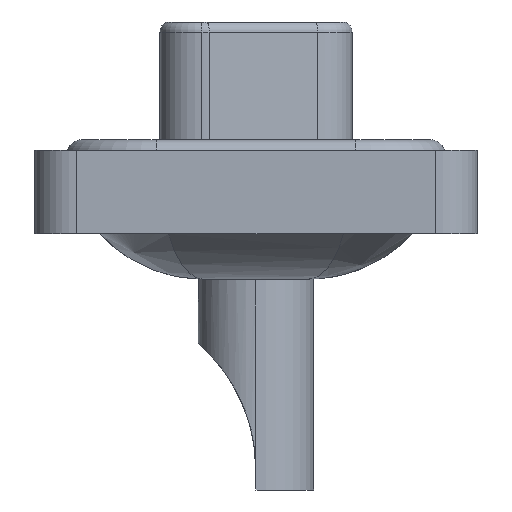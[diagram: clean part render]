
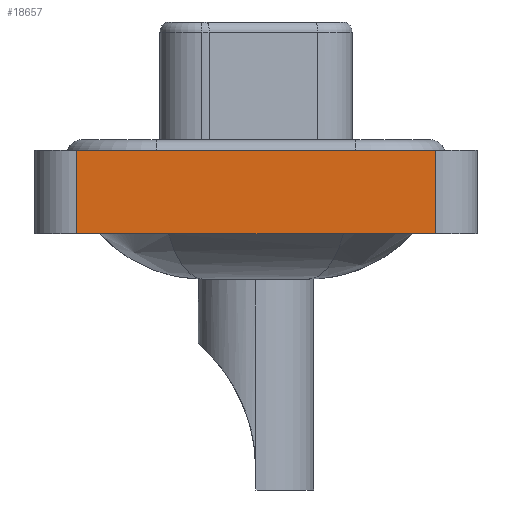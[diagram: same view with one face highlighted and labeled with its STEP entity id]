
A CAD part, left-side view. The second image highlights one B-rep face of the part: STEP entity #18657.
In plain terms, the highlighted planar face has unit normal (-1, 0, 0).
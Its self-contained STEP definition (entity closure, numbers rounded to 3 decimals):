
#525 = CARTESIAN_POINT ( 'NONE',  ( -7.3, 8.55, -3.6 ) ) ;
#1824 = DIRECTION ( 'NONE',  ( 0., 0., 1. ) ) ;
#2020 = VECTOR ( 'NONE', #8798, 1000. ) ;
#2289 = DIRECTION ( 'NONE',  ( 0., -1., 0. ) ) ;
#2310 = AXIS2_PLACEMENT_3D ( 'NONE', #18246, #2841, #11934 ) ;
#2841 = DIRECTION ( 'NONE',  ( -1., 0., 0. ) ) ;
#3316 = CARTESIAN_POINT ( 'NONE',  ( -7.3, -8.55, -3.6 ) ) ;
#5328 = LINE ( 'NONE', #16010, #2020 ) ;
#5745 = EDGE_CURVE ( 'NONE', #13799, #13626, #14313, .T. ) ;
#7313 = EDGE_CURVE ( 'NONE', #13799, #19292, #8191, .T. ) ;
#7655 = CARTESIAN_POINT ( 'NONE',  ( -7.3, 8.55, 0.4 ) ) ;
#8191 = LINE ( 'NONE', #15798, #13443 ) ;
#8519 = EDGE_CURVE ( 'NONE', #19292, #9419, #12498, .T. ) ;
#8798 = DIRECTION ( 'NONE',  ( 0., -1., 0. ) ) ;
#8835 = PLANE ( 'NONE',  #2310 ) ;
#9093 = EDGE_LOOP ( 'NONE', ( #17669, #11593, #18721, #11417 ) ) ;
#9419 = VERTEX_POINT ( 'NONE', #18462 ) ;
#9427 = DIRECTION ( 'NONE',  ( 0., 0., 1. ) ) ;
#9549 = VECTOR ( 'NONE', #9427, 1000. ) ;
#9996 = EDGE_CURVE ( 'NONE', #13626, #9419, #5328, .T. ) ;
#10046 = CARTESIAN_POINT ( 'NONE',  ( -7.3, 8.55, -3.6 ) ) ;
#11204 = CARTESIAN_POINT ( 'NONE',  ( -7.3, -8.55, -3.6 ) ) ;
#11417 = ORIENTED_EDGE ( 'NONE', *, *, #7313, .T. ) ;
#11593 = ORIENTED_EDGE ( 'NONE', *, *, #9996, .F. ) ;
#11934 = DIRECTION ( 'NONE',  ( 0., 0., 1. ) ) ;
#12498 = LINE ( 'NONE', #3316, #9549 ) ;
#13443 = VECTOR ( 'NONE', #2289, 1000. ) ;
#13626 = VERTEX_POINT ( 'NONE', #7655 ) ;
#13799 = VERTEX_POINT ( 'NONE', #10046 ) ;
#14313 = LINE ( 'NONE', #525, #17245 ) ;
#15798 = CARTESIAN_POINT ( 'NONE',  ( -7.3, -8.55, -3.6 ) ) ;
#16010 = CARTESIAN_POINT ( 'NONE',  ( -7.3, -8.55, 0.4 ) ) ;
#17245 = VECTOR ( 'NONE', #1824, 1000. ) ;
#17669 = ORIENTED_EDGE ( 'NONE', *, *, #8519, .T. ) ;
#18246 = CARTESIAN_POINT ( 'NONE',  ( -7.3, -8.55, -3.6 ) ) ;
#18462 = CARTESIAN_POINT ( 'NONE',  ( -7.3, -8.55, 0.4 ) ) ;
#18657 = ADVANCED_FACE ( 'NONE', ( #19533 ), #8835, .T. ) ;
#18721 = ORIENTED_EDGE ( 'NONE', *, *, #5745, .F. ) ;
#19292 = VERTEX_POINT ( 'NONE', #11204 ) ;
#19533 = FACE_OUTER_BOUND ( 'NONE', #9093, .T. ) ;
